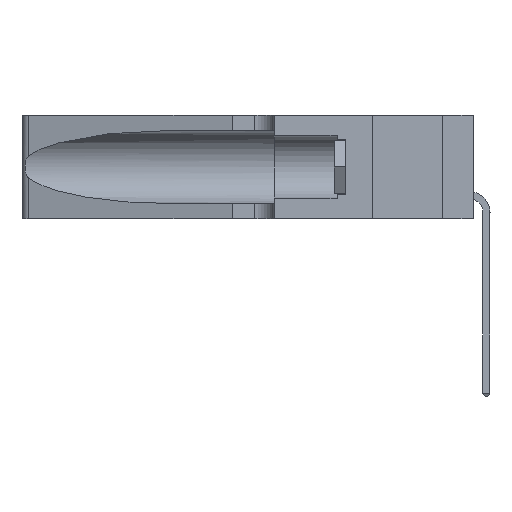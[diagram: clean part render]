
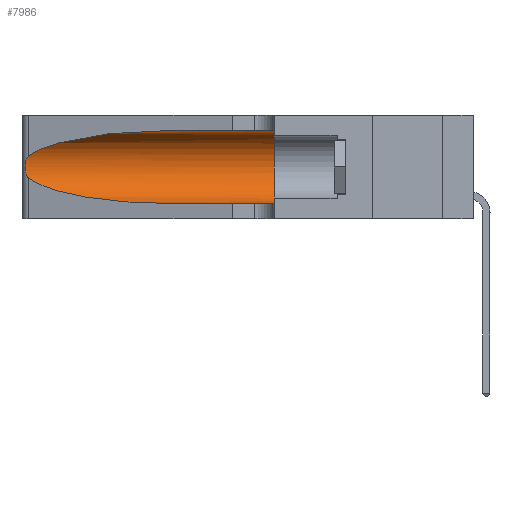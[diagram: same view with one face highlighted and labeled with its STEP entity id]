
A CAD part, left-side view. The second image highlights one B-rep face of the part: STEP entity #7986.
In plain terms, the highlighted cylindrical face has radius 3.308 mm (diameter 6.617 mm), a partial arc.
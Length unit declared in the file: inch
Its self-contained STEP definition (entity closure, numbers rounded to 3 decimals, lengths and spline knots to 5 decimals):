
#515 = LINE ( 'NONE', #18147, #37068 ) ;
#706 = EDGE_LOOP ( 'NONE', ( #886, #26570, #10638, #37936, #35907, #6227 ) ) ;
#886 = ORIENTED_EDGE ( 'NONE', *, *, #29714, .T. ) ;
#2004 = EDGE_CURVE ( 'NONE', #31460, #30341, #43810, .T. ) ;
#2854 = CARTESIAN_POINT ( 'NONE',  ( 0.1305, 0.72297, 0.05475 ) ) ;
#5403 = CARTESIAN_POINT ( 'NONE',  ( 0.1305, 0.35, 0.31525 ) ) ;
#6227 = ORIENTED_EDGE ( 'NONE', *, *, #25865, .F. ) ;
#6338 = CARTESIAN_POINT ( 'NONE',  ( 0.25639, 1.23184, 0.21858 ) ) ;
#6631 = AXIS2_PLACEMENT_3D ( 'NONE', #7179, #17671, #28225 ) ;
#6652 = CARTESIAN_POINT ( 'NONE',  ( 0.25787, 1.23484, 0.2124 ) ) ;
#7010 = CARTESIAN_POINT ( 'NONE',  ( 0.18966, 0.96281, 0.05475 ) ) ;
#7179 = CARTESIAN_POINT ( 'NONE',  ( 0.1305, 0.35, 0.185 ) ) ;
#7986 = ADVANCED_FACE ( 'NONE', ( #24677 ), #35236, .F. ) ;
#8802 = VERTEX_POINT ( 'NONE', #41065 ) ;
#9792 = VECTOR ( 'NONE', #14404, 39.37008 ) ;
#10011 = CARTESIAN_POINT ( 'NONE',  ( 0.2373, 1.15595, 0.28018 ) ) ;
#10167 = CARTESIAN_POINT ( 'NONE',  ( 0.25854, 1.2359, 0.20912 ) ) ;
#10363 = CARTESIAN_POINT ( 'NONE',  ( 0.1305, 0.72297, 0.05475 ) ) ;
#10638 = ORIENTED_EDGE ( 'NONE', *, *, #41121, .T. ) ;
#14072 = CARTESIAN_POINT ( 'NONE',  ( 0.25487, 1.22718, 0.14631 ) ) ;
#14404 = DIRECTION ( 'NONE',  ( 0., -1., 0. ) ) ;
#14973 = VERTEX_POINT ( 'NONE', #2854 ) ;
#16212 = CARTESIAN_POINT ( 'NONE',  ( 0.1305, 0.72297, 0.31525 ) ) ;
#17081 = CARTESIAN_POINT ( 'NONE',  ( 0.1305, 0.35, 0.05475 ) ) ;
#17278 = CARTESIAN_POINT ( 'NONE',  ( 0.1305, 0.72297, 0.31525 ) ) ;
#17294 = CARTESIAN_POINT ( 'NONE',  ( 0.26018, 1.23835, 0.19895 ) ) ;
#17422 = CARTESIAN_POINT ( 'NONE',  ( 0.25487, 1.22718, 0.22369 ) ) ;
#17671 = DIRECTION ( 'NONE',  ( 0., 1., 0. ) ) ;
#18147 = CARTESIAN_POINT ( 'NONE',  ( 0.1305, 1.61858, 0.05475 ) ) ;
#21269 = CARTESIAN_POINT ( 'NONE',  ( 0.1305, 1.61858, 0.31525 ) ) ;
#21433 = CARTESIAN_POINT ( 'NONE',  ( 0.26075, 1.23896, 0.178 ) ) ;
#21741 = CARTESIAN_POINT ( 'NONE',  ( 0.26075, 1.23896, 0.19203 ) ) ;
#21920 = LINE ( 'NONE', #21269, #9792 ) ;
#24265 = CARTESIAN_POINT ( 'NONE',  ( 0.18966, 0.96281, 0.31525 ) ) ;
#24497 = EDGE_CURVE ( 'NONE', #14973, #30341, #515, .T. ) ;
#24677 = FACE_OUTER_BOUND ( 'NONE', #706, .T. ) ;
#25016 = CARTESIAN_POINT ( 'NONE',  ( 0.25856, 1.23593, 0.16098 ) ) ;
#25049 =( BOUNDED_CURVE ( )  B_SPLINE_CURVE ( 3, ( #17278, #24265, #10011, #17422 ),
 .UNSPECIFIED., .F., .F. ) 
 B_SPLINE_CURVE_WITH_KNOTS ( ( 4, 4 ),
 ( 1.5708, 2.84003 ),
 .UNSPECIFIED. ) 
 CURVE ( )  GEOMETRIC_REPRESENTATION_ITEM ( )  RATIONAL_B_SPLINE_CURVE ( ( 1., 0.87, 0.87, 1. ) ) 
 REPRESENTATION_ITEM ( '' )  );
#25439 = DIRECTION ( 'NONE',  ( 0., -1., 0. ) ) ;
#25865 = EDGE_CURVE ( 'NONE', #40321, #31460, #21920, .T. ) ;
#26570 = ORIENTED_EDGE ( 'NONE', *, *, #28935, .T. ) ;
#28225 = DIRECTION ( 'NONE',  ( 0., 0., 1. ) ) ;
#28935 = EDGE_CURVE ( 'NONE', #41988, #8802, #36701, .T. ) ;
#28973 = CARTESIAN_POINT ( 'NONE',  ( 0.25487, 1.22718, 0.22369 ) ) ;
#29576 = CARTESIAN_POINT ( 'NONE',  ( 0.1305, 1.61858, 0.185 ) ) ;
#29714 = EDGE_CURVE ( 'NONE', #40321, #41988, #25049, .T. ) ;
#29892 =( BOUNDED_CURVE ( )  B_SPLINE_CURVE ( 3, ( #14072, #42102, #7010, #10363 ),
 .UNSPECIFIED., .F., .F. ) 
 B_SPLINE_CURVE_WITH_KNOTS ( ( 4, 4 ),
 ( 3.44316, 4.71239 ),
 .UNSPECIFIED. ) 
 CURVE ( )  GEOMETRIC_REPRESENTATION_ITEM ( )  RATIONAL_B_SPLINE_CURVE ( ( 1., 0.87, 0.87, 1. ) ) 
 REPRESENTATION_ITEM ( '' )  );
#30341 = VERTEX_POINT ( 'NONE', #17081 ) ;
#31114 = AXIS2_PLACEMENT_3D ( 'NONE', #29576, #33843, #44275 ) ;
#31460 = VERTEX_POINT ( 'NONE', #5403 ) ;
#33843 = DIRECTION ( 'NONE',  ( 0., -1., 0. ) ) ;
#35236 = CYLINDRICAL_SURFACE ( 'NONE', #31114, 0.13025 ) ;
#35416 = CARTESIAN_POINT ( 'NONE',  ( 0.25789, 1.23486, 0.15765 ) ) ;
#35703 = CARTESIAN_POINT ( 'NONE',  ( 0.25487, 1.22718, 0.14631 ) ) ;
#35907 = ORIENTED_EDGE ( 'NONE', *, *, #2004, .F. ) ;
#36701 = B_SPLINE_CURVE_WITH_KNOTS ( 'NONE', 3,
 ( #38646, #45276, #6338, #6652, #10167, #17294, #21741, #21433, #42752, #25016, #35416, #38938, #42468, #35703 ),
 .UNSPECIFIED., .F., .F.,
 ( 4, 2, 2, 2, 2, 2, 4 ),
 ( 0., 0.00027, 0.00053, 0.00107, 0.0016, 0.00187, 0.00214 ),
 .UNSPECIFIED. ) ;
#37068 = VECTOR ( 'NONE', #25439, 39.37008 ) ;
#37936 = ORIENTED_EDGE ( 'NONE', *, *, #24497, .T. ) ;
#38646 = CARTESIAN_POINT ( 'NONE',  ( 0.25487, 1.22718, 0.22369 ) ) ;
#38938 = CARTESIAN_POINT ( 'NONE',  ( 0.25639, 1.23186, 0.15144 ) ) ;
#40321 = VERTEX_POINT ( 'NONE', #16212 ) ;
#41065 = CARTESIAN_POINT ( 'NONE',  ( 0.25487, 1.22718, 0.14631 ) ) ;
#41121 = EDGE_CURVE ( 'NONE', #8802, #14973, #29892, .T. ) ;
#41988 = VERTEX_POINT ( 'NONE', #28973 ) ;
#42102 = CARTESIAN_POINT ( 'NONE',  ( 0.2373, 1.15595, 0.08982 ) ) ;
#42468 = CARTESIAN_POINT ( 'NONE',  ( 0.25555, 1.22993, 0.14849 ) ) ;
#42752 = CARTESIAN_POINT ( 'NONE',  ( 0.26017, 1.23833, 0.17102 ) ) ;
#43810 = CIRCLE ( 'NONE', #6631, 0.13025 ) ;
#44275 = DIRECTION ( 'NONE',  ( 0., 0., -1. ) ) ;
#45276 = CARTESIAN_POINT ( 'NONE',  ( 0.25555, 1.22994, 0.2215 ) ) ;
